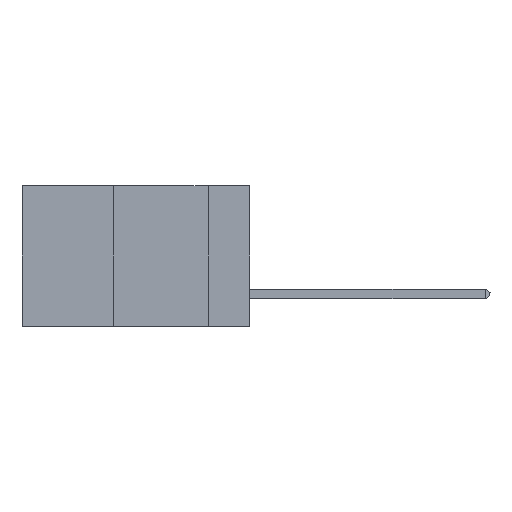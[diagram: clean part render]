
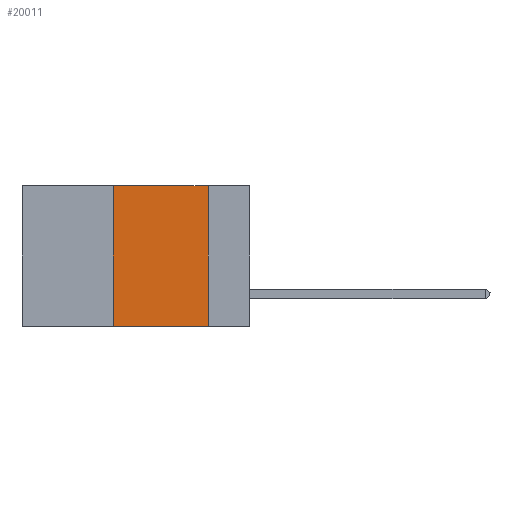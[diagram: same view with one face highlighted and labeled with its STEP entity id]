
A CAD part, left-side view. The second image highlights one B-rep face of the part: STEP entity #20011.
In plain terms, the highlighted planar face has unit normal (-1, 0, 0).
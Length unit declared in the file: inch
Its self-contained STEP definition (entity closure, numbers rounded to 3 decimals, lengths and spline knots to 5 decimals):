
#672 = DIRECTION ( 'NONE',  ( 0., 0., 1. ) ) ;
#1759 = DIRECTION ( 'NONE',  ( 0., 0., -1. ) ) ;
#2429 = EDGE_LOOP ( 'NONE', ( #20152, #18016, #23409, #26988 ) ) ;
#3405 = EDGE_CURVE ( 'NONE', #32891, #12138, #8548, .T. ) ;
#3824 = CARTESIAN_POINT ( 'NONE',  ( 0., 0.11, 0. ) ) ;
#4208 = VECTOR ( 'NONE', #27707, 39.37008 ) ;
#6047 = AXIS2_PLACEMENT_3D ( 'NONE', #30500, #30722, #20746 ) ;
#7470 = FACE_OUTER_BOUND ( 'NONE', #2429, .T. ) ;
#8548 = LINE ( 'NONE', #11429, #29598 ) ;
#8628 = DIRECTION ( 'NONE',  ( 0., -1., 0. ) ) ;
#9266 = LINE ( 'NONE', #17589, #10928 ) ;
#10440 = LINE ( 'NONE', #27940, #4208 ) ;
#10928 = VECTOR ( 'NONE', #1759, 39.37008 ) ;
#11429 = CARTESIAN_POINT ( 'NONE',  ( 0., 0.36, 0. ) ) ;
#11533 = CARTESIAN_POINT ( 'NONE',  ( 0., 0.6, -0.37 ) ) ;
#12067 = PLANE ( 'NONE',  #6047 ) ;
#12138 = VERTEX_POINT ( 'NONE', #23934 ) ;
#15609 = LINE ( 'NONE', #11533, #22646 ) ;
#16195 = EDGE_CURVE ( 'NONE', #32891, #21419, #15609, .T. ) ;
#17589 = CARTESIAN_POINT ( 'NONE',  ( 0., 0.11, 0. ) ) ;
#18016 = ORIENTED_EDGE ( 'NONE', *, *, #19357, .F. ) ;
#19357 = EDGE_CURVE ( 'NONE', #12138, #21849, #10440, .T. ) ;
#20011 = ADVANCED_FACE ( 'NONE', ( #7470 ), #12067, .F. ) ;
#20152 = ORIENTED_EDGE ( 'NONE', *, *, #28109, .F. ) ;
#20746 = DIRECTION ( 'NONE',  ( 0., 0., -1. ) ) ;
#21419 = VERTEX_POINT ( 'NONE', #22952 ) ;
#21849 = VERTEX_POINT ( 'NONE', #3824 ) ;
#22646 = VECTOR ( 'NONE', #8628, 39.37008 ) ;
#22952 = CARTESIAN_POINT ( 'NONE',  ( 0., 0.11, -0.37 ) ) ;
#23409 = ORIENTED_EDGE ( 'NONE', *, *, #3405, .F. ) ;
#23934 = CARTESIAN_POINT ( 'NONE',  ( 0., 0.36, 0. ) ) ;
#26988 = ORIENTED_EDGE ( 'NONE', *, *, #16195, .T. ) ;
#27707 = DIRECTION ( 'NONE',  ( 0., -1., 0. ) ) ;
#27940 = CARTESIAN_POINT ( 'NONE',  ( 0., 0.6, 0. ) ) ;
#28109 = EDGE_CURVE ( 'NONE', #21849, #21419, #9266, .T. ) ;
#29598 = VECTOR ( 'NONE', #672, 39.37008 ) ;
#30500 = CARTESIAN_POINT ( 'NONE',  ( 0., 0.6, 0. ) ) ;
#30722 = DIRECTION ( 'NONE',  ( 1., 0., 0. ) ) ;
#32891 = VERTEX_POINT ( 'NONE', #33237 ) ;
#33237 = CARTESIAN_POINT ( 'NONE',  ( 0., 0.36, -0.37 ) ) ;
